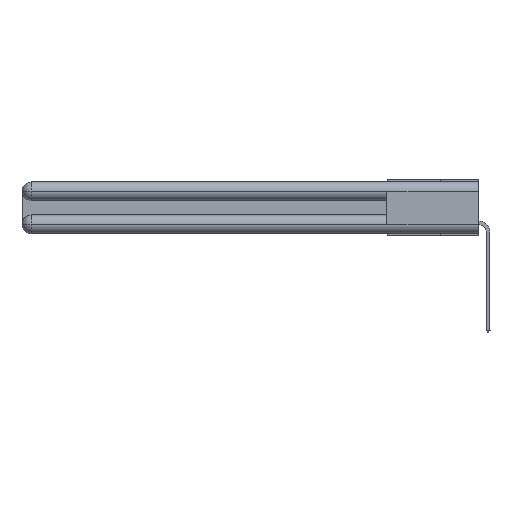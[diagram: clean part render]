
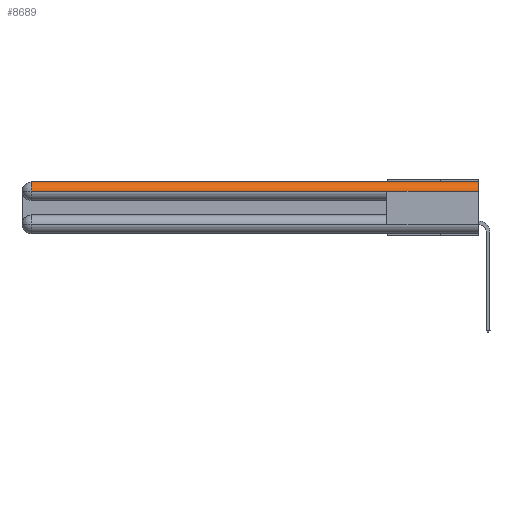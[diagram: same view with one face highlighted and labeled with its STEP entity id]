
A CAD part, left-side view. The second image highlights one B-rep face of the part: STEP entity #8689.
In plain terms, the highlighted cylindrical face has radius 1.562 mm (diameter 3.124 mm), a partial arc.
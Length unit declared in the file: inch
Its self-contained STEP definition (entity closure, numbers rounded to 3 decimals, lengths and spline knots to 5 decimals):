
#2125 = ORIENTED_EDGE ( 'NONE', *, *, #9606, .F. ) ;
#2411 = CIRCLE ( 'NONE', #4521, 0.0615 ) ;
#2781 = DIRECTION ( 'NONE',  ( 0., -1., 0. ) ) ;
#4120 = VERTEX_POINT ( 'NONE', #11121 ) ;
#4521 = AXIS2_PLACEMENT_3D ( 'NONE', #7778, #2781, #14711 ) ;
#5169 = CARTESIAN_POINT ( 'NONE',  ( 0.0615, 0., 0. ) ) ;
#5528 = CARTESIAN_POINT ( 'NONE',  ( 0.0615, 0., -0.0615 ) ) ;
#5598 = VECTOR ( 'NONE', #23673, 39.37008 ) ;
#5630 = VECTOR ( 'NONE', #27521, 39.37008 ) ;
#6407 = ORIENTED_EDGE ( 'NONE', *, *, #30046, .F. ) ;
#7660 = EDGE_CURVE ( 'NONE', #30244, #4120, #28314, .T. ) ;
#7778 = CARTESIAN_POINT ( 'NONE',  ( 0.0615, 2.94, -0.0615 ) ) ;
#7963 = DIRECTION ( 'NONE',  ( 1., 0., 0. ) ) ;
#8689 = ADVANCED_FACE ( 'NONE', ( #9206 ), #12859, .T. ) ;
#8801 = CARTESIAN_POINT ( 'NONE',  ( 0., 3., -0.0615 ) ) ;
#9206 = FACE_OUTER_BOUND ( 'NONE', #11629, .T. ) ;
#9502 = LINE ( 'NONE', #17445, #21923 ) ;
#9606 = EDGE_CURVE ( 'NONE', #16152, #18209, #26339, .T. ) ;
#9882 = DIRECTION ( 'NONE',  ( 0., 1., 0. ) ) ;
#11121 = CARTESIAN_POINT ( 'NONE',  ( 0., 0.6, -0.0615 ) ) ;
#11629 = EDGE_LOOP ( 'NONE', ( #15102, #21772, #25740, #6407, #2125 ) ) ;
#12650 = DIRECTION ( 'NONE',  ( 0., -1., 0. ) ) ;
#12859 = CYLINDRICAL_SURFACE ( 'NONE', #16855, 0.0615 ) ;
#13756 = CARTESIAN_POINT ( 'NONE',  ( 0.0615, 0., -0.0615 ) ) ;
#14024 = CARTESIAN_POINT ( 'NONE',  ( 0., 0., -0.0615 ) ) ;
#14677 = AXIS2_PLACEMENT_3D ( 'NONE', #5528, #12650, #7963 ) ;
#14711 = DIRECTION ( 'NONE',  ( 0., 0., 1. ) ) ;
#14735 = LINE ( 'NONE', #23570, #5598 ) ;
#15102 = ORIENTED_EDGE ( 'NONE', *, *, #25861, .F. ) ;
#15382 = CARTESIAN_POINT ( 'NONE',  ( 0.0615, 2.94, 0. ) ) ;
#16152 = VERTEX_POINT ( 'NONE', #5169 ) ;
#16855 = AXIS2_PLACEMENT_3D ( 'NONE', #13756, #9882, #18379 ) ;
#17445 = CARTESIAN_POINT ( 'NONE',  ( 0.0615, 0., 0. ) ) ;
#18209 = VERTEX_POINT ( 'NONE', #14024 ) ;
#18379 = DIRECTION ( 'NONE',  ( 0., 0., 1. ) ) ;
#18914 = EDGE_CURVE ( 'NONE', #30254, #30244, #2411, .T. ) ;
#20220 = DIRECTION ( 'NONE',  ( 0., -1., 0. ) ) ;
#21772 = ORIENTED_EDGE ( 'NONE', *, *, #18914, .T. ) ;
#21923 = VECTOR ( 'NONE', #20220, 39.37008 ) ;
#23570 = CARTESIAN_POINT ( 'NONE',  ( 0., 3., -0.0615 ) ) ;
#23673 = DIRECTION ( 'NONE',  ( 0., 1., 0. ) ) ;
#25740 = ORIENTED_EDGE ( 'NONE', *, *, #7660, .T. ) ;
#25861 = EDGE_CURVE ( 'NONE', #30254, #16152, #9502, .T. ) ;
#26339 = CIRCLE ( 'NONE', #14677, 0.0615 ) ;
#27331 = CARTESIAN_POINT ( 'NONE',  ( 0., 2.94, -0.0615 ) ) ;
#27521 = DIRECTION ( 'NONE',  ( 0., -1., 0. ) ) ;
#28314 = LINE ( 'NONE', #8801, #5630 ) ;
#30046 = EDGE_CURVE ( 'NONE', #18209, #4120, #14735, .T. ) ;
#30244 = VERTEX_POINT ( 'NONE', #27331 ) ;
#30254 = VERTEX_POINT ( 'NONE', #15382 ) ;
